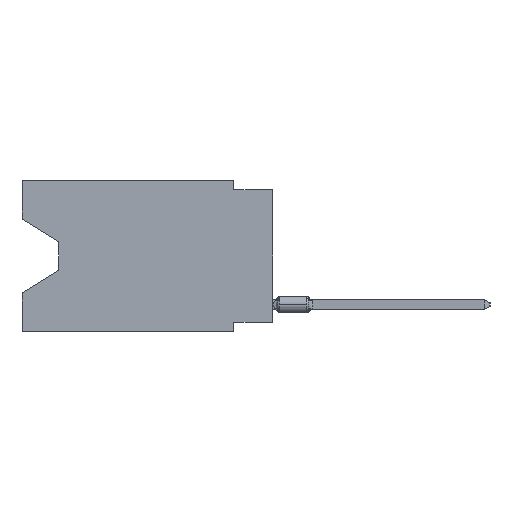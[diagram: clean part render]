
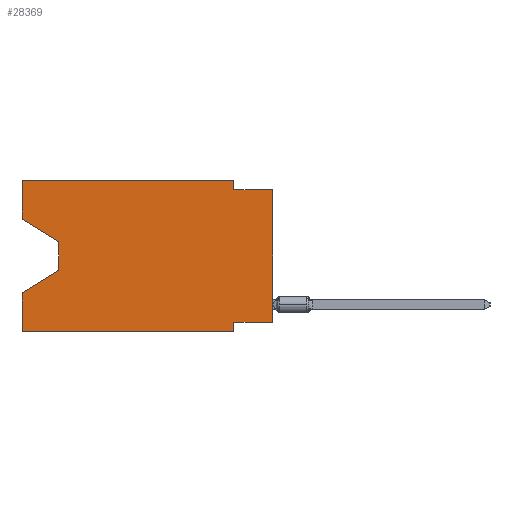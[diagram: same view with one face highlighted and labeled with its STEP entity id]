
A CAD part, left-side view. The second image highlights one B-rep face of the part: STEP entity #28369.
In plain terms, the highlighted planar face has unit normal (-1, 0, 0).
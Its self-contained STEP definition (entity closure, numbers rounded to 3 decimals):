
#161 = DIRECTION ( 'NONE',  ( 0., 0., 1. ) ) ;
#757 = VECTOR ( 'NONE', #40139, 1000. ) ;
#1183 = VECTOR ( 'NONE', #11588, 1000. ) ;
#1471 = VERTEX_POINT ( 'NONE', #14717 ) ;
#1652 = CARTESIAN_POINT ( 'NONE',  ( 0., 16.383, 0. ) ) ;
#1773 = VERTEX_POINT ( 'NONE', #58660 ) ;
#2169 = EDGE_CURVE ( 'NONE', #21879, #1773, #24530, .T. ) ;
#2607 = CARTESIAN_POINT ( 'NONE',  ( 0., 16.383, 0. ) ) ;
#2708 = AXIS2_PLACEMENT_3D ( 'NONE', #1652, #61019, #7411 ) ;
#3135 = VERTEX_POINT ( 'NONE', #20953 ) ;
#3197 = LINE ( 'NONE', #42055, #62831 ) ;
#4584 = VERTEX_POINT ( 'NONE', #35976 ) ;
#6722 = EDGE_CURVE ( 'NONE', #1471, #39634, #3197, .T. ) ;
#7411 = DIRECTION ( 'NONE',  ( 0., 0., -1. ) ) ;
#7434 = DIRECTION ( 'NONE',  ( 0., 0., 1. ) ) ;
#8178 = DIRECTION ( 'NONE',  ( 0., -1., 0. ) ) ;
#8944 = VECTOR ( 'NONE', #57720, 1000. ) ;
#9450 = EDGE_CURVE ( 'NONE', #4584, #1773, #29869, .T. ) ;
#10299 = ORIENTED_EDGE ( 'NONE', *, *, #49072, .T. ) ;
#11588 = DIRECTION ( 'NONE',  ( 0., 0., -1. ) ) ;
#13942 = CARTESIAN_POINT ( 'NONE',  ( 0., 0., 0. ) ) ;
#14129 = DIRECTION ( 'NONE',  ( 0., -1., 0. ) ) ;
#14433 = ORIENTED_EDGE ( 'NONE', *, *, #2169, .T. ) ;
#14717 = CARTESIAN_POINT ( 'NONE',  ( 0., 16.383, -2.546 ) ) ;
#16137 = ORIENTED_EDGE ( 'NONE', *, *, #9450, .F. ) ;
#18536 = LINE ( 'NONE', #38159, #8944 ) ;
#20355 = VECTOR ( 'NONE', #161, 1000. ) ;
#20953 = CARTESIAN_POINT ( 'NONE',  ( 0., 16.383, -7.36 ) ) ;
#21363 = ORIENTED_EDGE ( 'NONE', *, *, #29828, .F. ) ;
#21879 = VERTEX_POINT ( 'NONE', #36323 ) ;
#22502 = EDGE_CURVE ( 'NONE', #62268, #39094, #43053, .T. ) ;
#24061 = CARTESIAN_POINT ( 'NONE',  ( 0., 16.383, -9.906 ) ) ;
#24530 = LINE ( 'NONE', #13942, #20355 ) ;
#25701 = CARTESIAN_POINT ( 'NONE',  ( 0., 13.97, -4.013 ) ) ;
#27140 = LINE ( 'NONE', #36792, #60290 ) ;
#28369 = ADVANCED_FACE ( 'NONE', ( #35369 ), #31790, .F. ) ;
#28551 = CARTESIAN_POINT ( 'NONE',  ( 0., 16.383, 0. ) ) ;
#29828 = EDGE_CURVE ( 'NONE', #62268, #3135, #27140, .T. ) ;
#29869 = LINE ( 'NONE', #44031, #54861 ) ;
#30138 = ORIENTED_EDGE ( 'NONE', *, *, #6722, .T. ) ;
#30581 = VECTOR ( 'NONE', #7434, 1000. ) ;
#30983 = EDGE_CURVE ( 'NONE', #21879, #35973, #31652, .T. ) ;
#31467 = ORIENTED_EDGE ( 'NONE', *, *, #57375, .F. ) ;
#31652 = LINE ( 'NONE', #36806, #757 ) ;
#31790 = PLANE ( 'NONE',  #2708 ) ;
#32248 = VERTEX_POINT ( 'NONE', #28551 ) ;
#32578 = LINE ( 'NONE', #60625, #37885 ) ;
#32933 = ORIENTED_EDGE ( 'NONE', *, *, #41676, .F. ) ;
#33053 = ORIENTED_EDGE ( 'NONE', *, *, #30983, .F. ) ;
#33103 = CARTESIAN_POINT ( 'NONE',  ( 0., 13.97, -5.893 ) ) ;
#34042 = VECTOR ( 'NONE', #8178, 1000. ) ;
#34392 = DIRECTION ( 'NONE',  ( 0., -1., 0. ) ) ;
#35369 = FACE_OUTER_BOUND ( 'NONE', #56494, .T. ) ;
#35584 = CARTESIAN_POINT ( 'NONE',  ( 0., 2.54, 0. ) ) ;
#35973 = VERTEX_POINT ( 'NONE', #52386 ) ;
#35976 = CARTESIAN_POINT ( 'NONE',  ( 0., 2.54, -0.635 ) ) ;
#36001 = LINE ( 'NONE', #55580, #1183 ) ;
#36323 = CARTESIAN_POINT ( 'NONE',  ( 0., 0., -9.271 ) ) ;
#36764 = CARTESIAN_POINT ( 'NONE',  ( 0., 16.383, 0. ) ) ;
#36792 = CARTESIAN_POINT ( 'NONE',  ( 0., 16.383, 0. ) ) ;
#36793 = ORIENTED_EDGE ( 'NONE', *, *, #40874, .T. ) ;
#36806 = CARTESIAN_POINT ( 'NONE',  ( 0., 0., -9.271 ) ) ;
#37602 = DIRECTION ( 'NONE',  ( 0., 0.855, -0.519 ) ) ;
#37885 = VECTOR ( 'NONE', #62445, 1000. ) ;
#38159 = CARTESIAN_POINT ( 'NONE',  ( 0., 2.54, -9.906 ) ) ;
#38430 = EDGE_CURVE ( 'NONE', #46830, #4584, #32578, .T. ) ;
#39094 = VERTEX_POINT ( 'NONE', #45469 ) ;
#39634 = VERTEX_POINT ( 'NONE', #25701 ) ;
#40139 = DIRECTION ( 'NONE',  ( 0., 1., 0. ) ) ;
#40874 = EDGE_CURVE ( 'NONE', #39634, #42118, #36001, .T. ) ;
#41673 = ORIENTED_EDGE ( 'NONE', *, *, #38430, .F. ) ;
#41676 = EDGE_CURVE ( 'NONE', #32248, #46830, #52173, .T. ) ;
#42055 = CARTESIAN_POINT ( 'NONE',  ( 0., 16.383, -2.546 ) ) ;
#42118 = VERTEX_POINT ( 'NONE', #62355 ) ;
#43053 = LINE ( 'NONE', #44007, #54198 ) ;
#44007 = CARTESIAN_POINT ( 'NONE',  ( 0., 16.383, -9.906 ) ) ;
#44031 = CARTESIAN_POINT ( 'NONE',  ( 0., 0., -0.635 ) ) ;
#45469 = CARTESIAN_POINT ( 'NONE',  ( 0., 2.54, -9.906 ) ) ;
#45800 = DIRECTION ( 'NONE',  ( 0., 0., 1. ) ) ;
#46830 = VERTEX_POINT ( 'NONE', #35584 ) ;
#49072 = EDGE_CURVE ( 'NONE', #42118, #3135, #52388, .T. ) ;
#52173 = LINE ( 'NONE', #36764, #34042 ) ;
#52386 = CARTESIAN_POINT ( 'NONE',  ( 0., 2.54, -9.271 ) ) ;
#52388 = LINE ( 'NONE', #33103, #58112 ) ;
#52902 = ORIENTED_EDGE ( 'NONE', *, *, #22502, .T. ) ;
#54198 = VECTOR ( 'NONE', #14129, 1000. ) ;
#54861 = VECTOR ( 'NONE', #34392, 1000. ) ;
#55580 = CARTESIAN_POINT ( 'NONE',  ( 0., 13.97, -4.013 ) ) ;
#55864 = DIRECTION ( 'NONE',  ( 0., -0.855, -0.519 ) ) ;
#56494 = EDGE_LOOP ( 'NONE', ( #30138, #36793, #10299, #21363, #52902, #31467, #33053, #14433, #16137, #41673, #32933, #63482 ) ) ;
#57375 = EDGE_CURVE ( 'NONE', #35973, #39094, #18536, .T. ) ;
#57720 = DIRECTION ( 'NONE',  ( 0., 0., -1. ) ) ;
#58112 = VECTOR ( 'NONE', #37602, 1000. ) ;
#58660 = CARTESIAN_POINT ( 'NONE',  ( 0., 0., -0.635 ) ) ;
#59773 = EDGE_CURVE ( 'NONE', #1471, #32248, #62004, .T. ) ;
#60290 = VECTOR ( 'NONE', #45800, 1000. ) ;
#60625 = CARTESIAN_POINT ( 'NONE',  ( 0., 2.54, 0. ) ) ;
#61019 = DIRECTION ( 'NONE',  ( 1., 0., 0. ) ) ;
#62004 = LINE ( 'NONE', #2607, #30581 ) ;
#62268 = VERTEX_POINT ( 'NONE', #24061 ) ;
#62355 = CARTESIAN_POINT ( 'NONE',  ( 0., 13.97, -5.893 ) ) ;
#62445 = DIRECTION ( 'NONE',  ( 0., 0., -1. ) ) ;
#62831 = VECTOR ( 'NONE', #55864, 1000. ) ;
#63482 = ORIENTED_EDGE ( 'NONE', *, *, #59773, .F. ) ;
